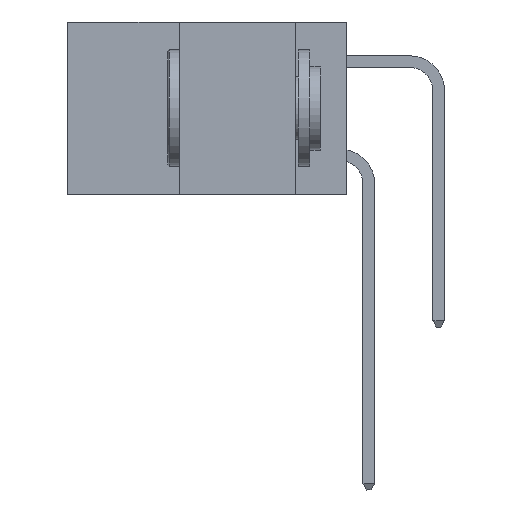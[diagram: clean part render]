
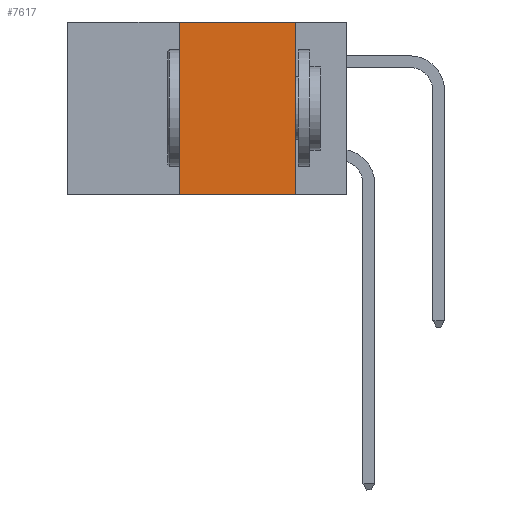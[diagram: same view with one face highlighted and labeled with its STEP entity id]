
A CAD part, left-side view. The second image highlights one B-rep face of the part: STEP entity #7617.
In plain terms, the highlighted planar face has unit normal (-1, 0, 0).
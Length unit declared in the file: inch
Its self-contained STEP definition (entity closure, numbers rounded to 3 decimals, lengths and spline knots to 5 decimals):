
#97 = DIRECTION ( 'NONE',  ( 0., -1., 0. ) ) ;
#1085 = VECTOR ( 'NONE', #97, 39.37008 ) ;
#1273 = CARTESIAN_POINT ( 'NONE',  ( 0., 0.36, -0.37 ) ) ;
#2548 = LINE ( 'NONE', #4914, #7309 ) ;
#3096 = CARTESIAN_POINT ( 'NONE',  ( 0., 0.36, 0. ) ) ;
#4009 = VECTOR ( 'NONE', #7437, 39.37008 ) ;
#4433 = VECTOR ( 'NONE', #4509, 39.37008 ) ;
#4509 = DIRECTION ( 'NONE',  ( 0., 0., 1. ) ) ;
#4914 = CARTESIAN_POINT ( 'NONE',  ( 0., 0.11, 0. ) ) ;
#5087 = CARTESIAN_POINT ( 'NONE',  ( 0., 0.6, 0. ) ) ;
#5214 = EDGE_CURVE ( 'NONE', #16874, #16042, #19310, .T. ) ;
#6078 = FACE_OUTER_BOUND ( 'NONE', #24145, .T. ) ;
#7309 = VECTOR ( 'NONE', #10753, 39.37008 ) ;
#7437 = DIRECTION ( 'NONE',  ( 0., -1., 0. ) ) ;
#7617 = ADVANCED_FACE ( 'NONE', ( #6078 ), #10924, .F. ) ;
#8819 = VERTEX_POINT ( 'NONE', #14513 ) ;
#9266 = CARTESIAN_POINT ( 'NONE',  ( 0., 0.6, -0.37 ) ) ;
#10058 = ORIENTED_EDGE ( 'NONE', *, *, #17263, .F. ) ;
#10222 = LINE ( 'NONE', #10368, #4433 ) ;
#10368 = CARTESIAN_POINT ( 'NONE',  ( 0., 0.36, 0. ) ) ;
#10753 = DIRECTION ( 'NONE',  ( 0., 0., -1. ) ) ;
#10924 = PLANE ( 'NONE',  #20544 ) ;
#11976 = CARTESIAN_POINT ( 'NONE',  ( 0., 0.6, 0. ) ) ;
#12165 = ORIENTED_EDGE ( 'NONE', *, *, #19042, .F. ) ;
#12869 = DIRECTION ( 'NONE',  ( 0., 0., -1. ) ) ;
#14513 = CARTESIAN_POINT ( 'NONE',  ( 0., 0.11, 0. ) ) ;
#14625 = CARTESIAN_POINT ( 'NONE',  ( 0., 0.11, -0.37 ) ) ;
#15774 = ORIENTED_EDGE ( 'NONE', *, *, #5214, .T. ) ;
#16035 = EDGE_CURVE ( 'NONE', #8819, #16042, #2548, .T. ) ;
#16042 = VERTEX_POINT ( 'NONE', #14625 ) ;
#16874 = VERTEX_POINT ( 'NONE', #1273 ) ;
#17263 = EDGE_CURVE ( 'NONE', #16874, #18113, #10222, .T. ) ;
#18113 = VERTEX_POINT ( 'NONE', #3096 ) ;
#19042 = EDGE_CURVE ( 'NONE', #18113, #8819, #22200, .T. ) ;
#19310 = LINE ( 'NONE', #9266, #4009 ) ;
#20544 = AXIS2_PLACEMENT_3D ( 'NONE', #5087, #24035, #12869 ) ;
#20982 = ORIENTED_EDGE ( 'NONE', *, *, #16035, .F. ) ;
#22200 = LINE ( 'NONE', #11976, #1085 ) ;
#24035 = DIRECTION ( 'NONE',  ( 1., 0., 0. ) ) ;
#24145 = EDGE_LOOP ( 'NONE', ( #20982, #12165, #10058, #15774 ) ) ;
